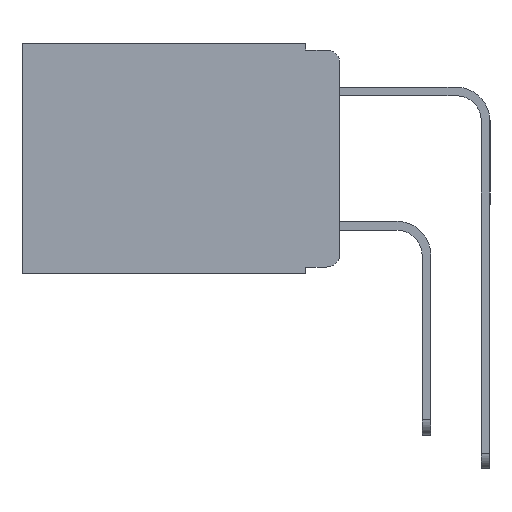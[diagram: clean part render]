
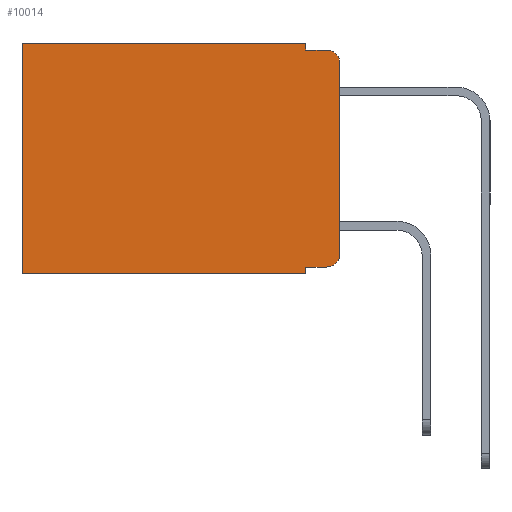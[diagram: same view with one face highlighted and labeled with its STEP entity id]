
A CAD part, left-side view. The second image highlights one B-rep face of the part: STEP entity #10014.
In plain terms, the highlighted planar face has unit normal (-1, 0, 0).
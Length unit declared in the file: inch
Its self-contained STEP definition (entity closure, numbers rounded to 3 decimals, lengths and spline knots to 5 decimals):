
#217 = CARTESIAN_POINT ( 'NONE',  ( 0.298, 0.473, -0.343 ) ) ;
#261 = CARTESIAN_POINT ( 'NONE',  ( 0.298, 0., 0. ) ) ;
#318 = CARTESIAN_POINT ( 'NONE',  ( 0.298, 0., -0.03 ) ) ;
#348 = ORIENTED_EDGE ( 'NONE', *, *, #9348, .T. ) ;
#749 = PLANE ( 'NONE',  #12170 ) ;
#750 = ORIENTED_EDGE ( 'NONE', *, *, #1917, .F. ) ;
#1176 = EDGE_CURVE ( 'NONE', #7260, #10157, #1994, .T. ) ;
#1555 = AXIS2_PLACEMENT_3D ( 'NONE', #12271, #8838, #7222 ) ;
#1654 = DIRECTION ( 'NONE',  ( 0., -1., 0. ) ) ;
#1779 = DIRECTION ( 'NONE',  ( 0., 0., -1. ) ) ;
#1830 = CARTESIAN_POINT ( 'NONE',  ( 0.298, 0.051, -0.333 ) ) ;
#1862 = ORIENTED_EDGE ( 'NONE', *, *, #7920, .T. ) ;
#1917 = EDGE_CURVE ( 'NONE', #6608, #11277, #7141, .T. ) ;
#1994 = LINE ( 'NONE', #6763, #11768 ) ;
#1998 = EDGE_LOOP ( 'NONE', ( #750, #1862, #11931, #9804, #10418, #4737, #8633, #10696, #348, #12110 ) ) ;
#2175 = CARTESIAN_POINT ( 'NONE',  ( 0.298, 0.051, -0.01 ) ) ;
#2195 = CARTESIAN_POINT ( 'NONE',  ( 0.298, 0., 0. ) ) ;
#2732 = DIRECTION ( 'NONE',  ( 0., 1., 0. ) ) ;
#2846 = CARTESIAN_POINT ( 'NONE',  ( 0.298, 0.051, 0. ) ) ;
#2859 = EDGE_CURVE ( 'NONE', #11180, #10157, #6124, .T. ) ;
#3132 = VERTEX_POINT ( 'NONE', #10185 ) ;
#3176 = VERTEX_POINT ( 'NONE', #2175 ) ;
#3908 = DIRECTION ( 'NONE',  ( 0., 0., -1. ) ) ;
#4401 = DIRECTION ( 'NONE',  ( 0., 0., -1. ) ) ;
#4737 = ORIENTED_EDGE ( 'NONE', *, *, #1176, .T. ) ;
#4997 = LINE ( 'NONE', #261, #12318 ) ;
#5094 = VERTEX_POINT ( 'NONE', #1830 ) ;
#5329 = VECTOR ( 'NONE', #7171, 39.37008 ) ;
#5516 = LINE ( 'NONE', #9357, #10392 ) ;
#5541 = VERTEX_POINT ( 'NONE', #6752 ) ;
#5948 = CARTESIAN_POINT ( 'NONE',  ( 0.298, 0., -0.343 ) ) ;
#6007 = CARTESIAN_POINT ( 'NONE',  ( 0.298, 0.051, -0.01 ) ) ;
#6124 = LINE ( 'NONE', #5948, #8294 ) ;
#6242 = CARTESIAN_POINT ( 'NONE',  ( 0.298, 0.02, -0.03 ) ) ;
#6316 = DIRECTION ( 'NONE',  ( 0., 1., 0. ) ) ;
#6528 = VERTEX_POINT ( 'NONE', #10267 ) ;
#6608 = VERTEX_POINT ( 'NONE', #318 ) ;
#6752 = CARTESIAN_POINT ( 'NONE',  ( 0.298, 0.02, -0.01 ) ) ;
#6763 = CARTESIAN_POINT ( 'NONE',  ( 0.298, 0.473, 0. ) ) ;
#6954 = CARTESIAN_POINT ( 'NONE',  ( 0.298, 0.473, 0. ) ) ;
#7141 = LINE ( 'NONE', #2195, #9214 ) ;
#7167 = CARTESIAN_POINT ( 'NONE',  ( 0.298, 0.051, -0.343 ) ) ;
#7171 = DIRECTION ( 'NONE',  ( 0., 0., -1. ) ) ;
#7222 = DIRECTION ( 'NONE',  ( 0., 0., -1. ) ) ;
#7260 = VERTEX_POINT ( 'NONE', #6954 ) ;
#7354 = EDGE_CURVE ( 'NONE', #5094, #11180, #5516, .T. ) ;
#7688 = DIRECTION ( 'NONE',  ( -1., 0., 0. ) ) ;
#7691 = DIRECTION ( 'NONE',  ( 1., 0., 0. ) ) ;
#7735 = VECTOR ( 'NONE', #1654, 39.37008 ) ;
#7739 = AXIS2_PLACEMENT_3D ( 'NONE', #6242, #7688, #12145 ) ;
#7799 = CARTESIAN_POINT ( 'NONE',  ( 0.298, 0.051, -0.333 ) ) ;
#7858 = LINE ( 'NONE', #2846, #5329 ) ;
#7920 = EDGE_CURVE ( 'NONE', #6608, #5541, #9549, .T. ) ;
#8089 = EDGE_CURVE ( 'NONE', #3132, #11277, #8177, .T. ) ;
#8177 = CIRCLE ( 'NONE', #1555, 0.02 ) ;
#8294 = VECTOR ( 'NONE', #2732, 39.37008 ) ;
#8466 = EDGE_CURVE ( 'NONE', #3176, #5541, #11084, .T. ) ;
#8633 = ORIENTED_EDGE ( 'NONE', *, *, #2859, .F. ) ;
#8729 = VECTOR ( 'NONE', #8903, 39.37008 ) ;
#8838 = DIRECTION ( 'NONE',  ( -1., 0., 0. ) ) ;
#8903 = DIRECTION ( 'NONE',  ( 0., -1., 0. ) ) ;
#9060 = CARTESIAN_POINT ( 'NONE',  ( 0.298, 0., -0.313 ) ) ;
#9214 = VECTOR ( 'NONE', #3908, 39.37008 ) ;
#9348 = EDGE_CURVE ( 'NONE', #5094, #3132, #10102, .T. ) ;
#9357 = CARTESIAN_POINT ( 'NONE',  ( 0.298, 0.051, 0. ) ) ;
#9549 = CIRCLE ( 'NONE', #7739, 0.02 ) ;
#9624 = EDGE_CURVE ( 'NONE', #6528, #3176, #7858, .T. ) ;
#9804 = ORIENTED_EDGE ( 'NONE', *, *, #9624, .F. ) ;
#10014 = ADVANCED_FACE ( 'NONE', ( #12194 ), #749, .F. ) ;
#10102 = LINE ( 'NONE', #7799, #7735 ) ;
#10157 = VERTEX_POINT ( 'NONE', #217 ) ;
#10185 = CARTESIAN_POINT ( 'NONE',  ( 0.298, 0.02, -0.333 ) ) ;
#10194 = EDGE_CURVE ( 'NONE', #6528, #7260, #4997, .T. ) ;
#10195 = DIRECTION ( 'NONE',  ( 0., 0., -1. ) ) ;
#10267 = CARTESIAN_POINT ( 'NONE',  ( 0.298, 0.051, 0. ) ) ;
#10392 = VECTOR ( 'NONE', #4401, 39.37008 ) ;
#10418 = ORIENTED_EDGE ( 'NONE', *, *, #10194, .T. ) ;
#10696 = ORIENTED_EDGE ( 'NONE', *, *, #7354, .F. ) ;
#11084 = LINE ( 'NONE', #6007, #8729 ) ;
#11180 = VERTEX_POINT ( 'NONE', #7167 ) ;
#11277 = VERTEX_POINT ( 'NONE', #9060 ) ;
#11287 = CARTESIAN_POINT ( 'NONE',  ( 0.298, 0., 0. ) ) ;
#11768 = VECTOR ( 'NONE', #10195, 39.37008 ) ;
#11931 = ORIENTED_EDGE ( 'NONE', *, *, #8466, .F. ) ;
#12110 = ORIENTED_EDGE ( 'NONE', *, *, #8089, .T. ) ;
#12145 = DIRECTION ( 'NONE',  ( 0., 0., -1. ) ) ;
#12170 = AXIS2_PLACEMENT_3D ( 'NONE', #11287, #7691, #1779 ) ;
#12194 = FACE_OUTER_BOUND ( 'NONE', #1998, .T. ) ;
#12271 = CARTESIAN_POINT ( 'NONE',  ( 0.298, 0.02, -0.313 ) ) ;
#12318 = VECTOR ( 'NONE', #6316, 39.37008 ) ;
